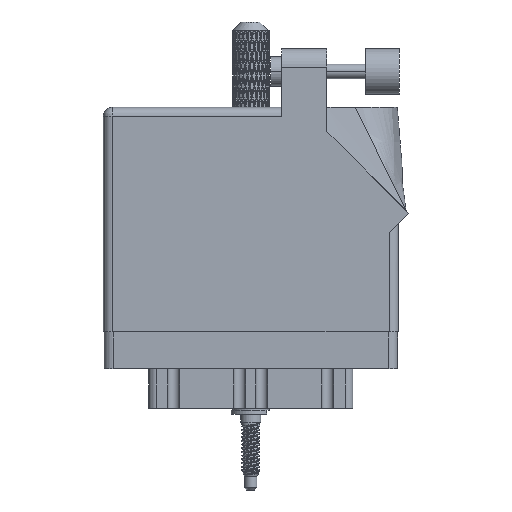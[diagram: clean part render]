
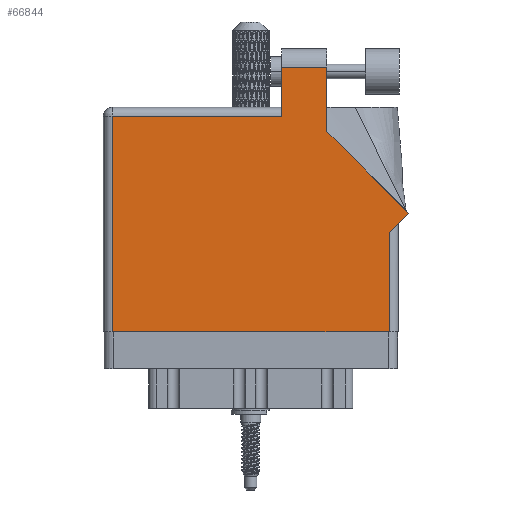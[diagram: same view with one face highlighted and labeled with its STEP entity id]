
A CAD part, front view. The second image highlights one B-rep face of the part: STEP entity #66844.
In plain terms, the highlighted face is planar.
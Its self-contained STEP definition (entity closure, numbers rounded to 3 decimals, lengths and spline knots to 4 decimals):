
#2007 = VECTOR ( 'NONE', #85959, 39.3701 ) ;
#6287 = VERTEX_POINT ( 'NONE', #37618 ) ;
#7535 = EDGE_CURVE ( 'NONE', #83016, #6287, #66727, .T. ) ;
#8743 = EDGE_LOOP ( 'NONE', ( #52733, #48691, #27627, #32275, #18256, #48839, #89350, #24870, #13340 ) ) ;
#9030 = VERTEX_POINT ( 'NONE', #62200 ) ;
#9123 = DIRECTION ( 'NONE',  ( 0., -1., 0. ) ) ;
#13340 = ORIENTED_EDGE ( 'NONE', *, *, #85253, .T. ) ;
#13959 = CARTESIAN_POINT ( 'NONE',  ( 2.0807, 0.8077, 0. ) ) ;
#14228 = CARTESIAN_POINT ( 'NONE',  ( 1.217, 1.805, 0. ) ) ;
#15754 = DIRECTION ( 'NONE',  ( 0., 0., -1. ) ) ;
#16889 = VECTOR ( 'NONE', #9123, 39.3701 ) ;
#18256 = ORIENTED_EDGE ( 'NONE', *, *, #19766, .T. ) ;
#19766 = EDGE_CURVE ( 'NONE', #71836, #9030, #65668, .T. ) ;
#19770 = CARTESIAN_POINT ( 'NONE',  ( 1.524, 1.805, 0. ) ) ;
#19843 = DIRECTION ( 'NONE',  ( 1., 0., 0. ) ) ;
#21875 = VERTEX_POINT ( 'NONE', #13959 ) ;
#24870 = ORIENTED_EDGE ( 'NONE', *, *, #55966, .T. ) ;
#27627 = ORIENTED_EDGE ( 'NONE', *, *, #7535, .T. ) ;
#28547 = DIRECTION ( 'NONE',  ( 0.707, 0.707, 0. ) ) ;
#28885 = CARTESIAN_POINT ( 'NONE',  ( 2.0807, 0.8077, 0. ) ) ;
#30398 = LINE ( 'NONE', #63178, #37593 ) ;
#30540 = DIRECTION ( 'NONE',  ( -1., 0., 0. ) ) ;
#31892 = CARTESIAN_POINT ( 'NONE',  ( 1.524, 1.3644, 0. ) ) ;
#32275 = ORIENTED_EDGE ( 'NONE', *, *, #99441, .T. ) ;
#33740 = VERTEX_POINT ( 'NONE', #81205 ) ;
#34114 = VERTEX_POINT ( 'NONE', #48893 ) ;
#37593 = VECTOR ( 'NONE', #38357, 39.3701 ) ;
#37618 = CARTESIAN_POINT ( 'NONE',  ( 1.217, 1.468, 0. ) ) ;
#38357 = DIRECTION ( 'NONE',  ( 0., 1., 0. ) ) ;
#40055 = CARTESIAN_POINT ( 'NONE',  ( 0., 1.53, 0. ) ) ;
#40178 = EDGE_CURVE ( 'NONE', #75632, #83016, #77664, .T. ) ;
#40846 = CARTESIAN_POINT ( 'NONE',  ( 1.217, 1.53, 0. ) ) ;
#41513 = EDGE_CURVE ( 'NONE', #9030, #58973, #101733, .T. ) ;
#42030 = EDGE_CURVE ( 'NONE', #33740, #75632, #73120, .T. ) ;
#46325 = LINE ( 'NONE', #102878, #2007 ) ;
#48691 = ORIENTED_EDGE ( 'NONE', *, *, #40178, .T. ) ;
#48839 = ORIENTED_EDGE ( 'NONE', *, *, #41513, .T. ) ;
#48893 = CARTESIAN_POINT ( 'NONE',  ( 1.948, 0.675, 0. ) ) ;
#51151 = LINE ( 'NONE', #28885, #86311 ) ;
#51409 = AXIS2_PLACEMENT_3D ( 'NONE', #40055, #15754, #30540 ) ;
#52612 = EDGE_CURVE ( 'NONE', #58973, #34114, #30398, .T. ) ;
#52733 = ORIENTED_EDGE ( 'NONE', *, *, #42030, .T. ) ;
#55966 = EDGE_CURVE ( 'NONE', #34114, #21875, #60288, .T. ) ;
#58973 = VERTEX_POINT ( 'NONE', #70701 ) ;
#60288 = LINE ( 'NONE', #67728, #88446 ) ;
#62200 = CARTESIAN_POINT ( 'NONE',  ( 0.062, 0., 0. ) ) ;
#62318 = DIRECTION ( 'NONE',  ( -1., 0., 0. ) ) ;
#63178 = CARTESIAN_POINT ( 'NONE',  ( 1.948, 0.737, 0. ) ) ;
#63938 = CARTESIAN_POINT ( 'NONE',  ( 1.217, 1.805, 0. ) ) ;
#64680 = DIRECTION ( 'NONE',  ( 0., 1., 0. ) ) ;
#64686 = CARTESIAN_POINT ( 'NONE',  ( 0.062, 1.468, 0. ) ) ;
#65668 = LINE ( 'NONE', #82574, #16889 ) ;
#66727 = LINE ( 'NONE', #40846, #100558 ) ;
#66844 = ADVANCED_FACE ( 'NONE', ( #88666 ), #71760, .F. ) ;
#67728 = CARTESIAN_POINT ( 'NONE',  ( 2.01, 0.737, 0. ) ) ;
#69067 = VECTOR ( 'NONE', #62318, 39.3701 ) ;
#70701 = CARTESIAN_POINT ( 'NONE',  ( 1.948, 0., 0. ) ) ;
#71760 = PLANE ( 'NONE',  #51409 ) ;
#71836 = VERTEX_POINT ( 'NONE', #64686 ) ;
#73120 = LINE ( 'NONE', #31892, #74218 ) ;
#74218 = VECTOR ( 'NONE', #64680, 39.3701 ) ;
#75632 = VERTEX_POINT ( 'NONE', #19770 ) ;
#77664 = LINE ( 'NONE', #14228, #69067 ) ;
#81003 = VECTOR ( 'NONE', #19843, 39.3701 ) ;
#81205 = CARTESIAN_POINT ( 'NONE',  ( 1.524, 1.3644, 0. ) ) ;
#82574 = CARTESIAN_POINT ( 'NONE',  ( 0.062, 0., 0. ) ) ;
#83016 = VERTEX_POINT ( 'NONE', #63938 ) ;
#83406 = DIRECTION ( 'NONE',  ( -0.707, 0.707, 0. ) ) ;
#85253 = EDGE_CURVE ( 'NONE', #21875, #33740, #51151, .T. ) ;
#85959 = DIRECTION ( 'NONE',  ( -1., 0., 0. ) ) ;
#86311 = VECTOR ( 'NONE', #83406, 39.3701 ) ;
#88446 = VECTOR ( 'NONE', #28547, 39.3701 ) ;
#88666 = FACE_OUTER_BOUND ( 'NONE', #8743, .T. ) ;
#89350 = ORIENTED_EDGE ( 'NONE', *, *, #52612, .T. ) ;
#94318 = CARTESIAN_POINT ( 'NONE',  ( 0., 0., 0. ) ) ;
#97382 = DIRECTION ( 'NONE',  ( 0., -1., 0. ) ) ;
#99441 = EDGE_CURVE ( 'NONE', #6287, #71836, #46325, .T. ) ;
#100558 = VECTOR ( 'NONE', #97382, 39.3701 ) ;
#101733 = LINE ( 'NONE', #94318, #81003 ) ;
#102878 = CARTESIAN_POINT ( 'NONE',  ( 0., 1.468, 0. ) ) ;
